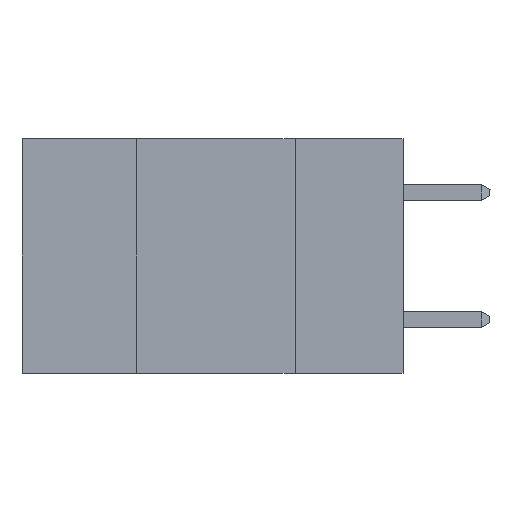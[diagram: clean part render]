
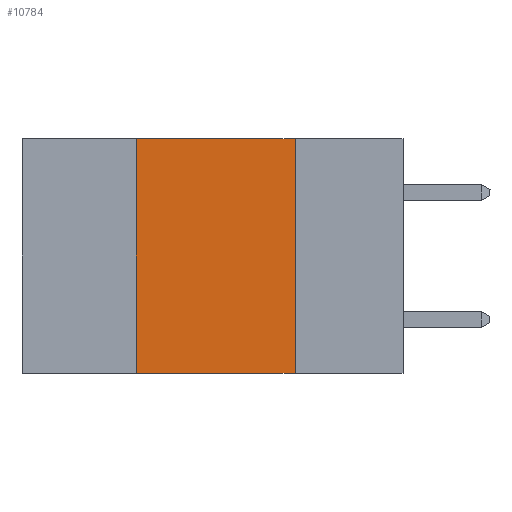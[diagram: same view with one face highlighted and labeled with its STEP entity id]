
A CAD part, left-side view. The second image highlights one B-rep face of the part: STEP entity #10784.
In plain terms, the highlighted planar face has unit normal (-1, 0, 0).
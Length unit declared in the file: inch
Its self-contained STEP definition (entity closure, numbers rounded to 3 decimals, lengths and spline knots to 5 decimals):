
#3 = VERTEX_POINT ( 'NONE', #3043 ) ;
#73 = CARTESIAN_POINT ( 'NONE',  ( 0., 0.17, 0. ) ) ;
#2201 = CARTESIAN_POINT ( 'NONE',  ( 0., 0.17, 0. ) ) ;
#2380 = CARTESIAN_POINT ( 'NONE',  ( 0., 0.6, 0. ) ) ;
#3043 = CARTESIAN_POINT ( 'NONE',  ( 0., 0.42, -0.37 ) ) ;
#3263 = DIRECTION ( 'NONE',  ( 0., 0., -1. ) ) ;
#3389 = DIRECTION ( 'NONE',  ( 0., 0., -1. ) ) ;
#3526 = VECTOR ( 'NONE', #5571, 39.37008 ) ;
#4343 = ORIENTED_EDGE ( 'NONE', *, *, #10769, .T. ) ;
#4359 = CARTESIAN_POINT ( 'NONE',  ( 0., 0.6, -0.37 ) ) ;
#4463 = VERTEX_POINT ( 'NONE', #10643 ) ;
#4992 = AXIS2_PLACEMENT_3D ( 'NONE', #7992, #10314, #3263 ) ;
#5478 = LINE ( 'NONE', #4359, #3526 ) ;
#5571 = DIRECTION ( 'NONE',  ( 0., -1., 0. ) ) ;
#5648 = LINE ( 'NONE', #2380, #14379 ) ;
#6502 = DIRECTION ( 'NONE',  ( 0., 0., 1. ) ) ;
#6694 = CARTESIAN_POINT ( 'NONE',  ( 0., 0.42, 0. ) ) ;
#7917 = EDGE_CURVE ( 'NONE', #3, #12047, #13660, .T. ) ;
#7992 = CARTESIAN_POINT ( 'NONE',  ( 0., 0.6, 0. ) ) ;
#8016 = VECTOR ( 'NONE', #6502, 39.37008 ) ;
#8285 = ORIENTED_EDGE ( 'NONE', *, *, #14298, .F. ) ;
#9071 = VERTEX_POINT ( 'NONE', #73 ) ;
#9914 = VECTOR ( 'NONE', #3389, 39.37008 ) ;
#10314 = DIRECTION ( 'NONE',  ( 1., 0., 0. ) ) ;
#10516 = ORIENTED_EDGE ( 'NONE', *, *, #13665, .F. ) ;
#10632 = DIRECTION ( 'NONE',  ( 0., -1., 0. ) ) ;
#10643 = CARTESIAN_POINT ( 'NONE',  ( 0., 0.17, -0.37 ) ) ;
#10769 = EDGE_CURVE ( 'NONE', #3, #4463, #5478, .T. ) ;
#10784 = ADVANCED_FACE ( 'NONE', ( #12483 ), #13611, .F. ) ;
#11949 = EDGE_LOOP ( 'NONE', ( #10516, #8285, #14442, #4343 ) ) ;
#12047 = VERTEX_POINT ( 'NONE', #6694 ) ;
#12483 = FACE_OUTER_BOUND ( 'NONE', #11949, .T. ) ;
#12918 = LINE ( 'NONE', #2201, #9914 ) ;
#13372 = CARTESIAN_POINT ( 'NONE',  ( 0., 0.42, 0. ) ) ;
#13611 = PLANE ( 'NONE',  #4992 ) ;
#13660 = LINE ( 'NONE', #13372, #8016 ) ;
#13665 = EDGE_CURVE ( 'NONE', #9071, #4463, #12918, .T. ) ;
#14298 = EDGE_CURVE ( 'NONE', #12047, #9071, #5648, .T. ) ;
#14379 = VECTOR ( 'NONE', #10632, 39.37008 ) ;
#14442 = ORIENTED_EDGE ( 'NONE', *, *, #7917, .F. ) ;
